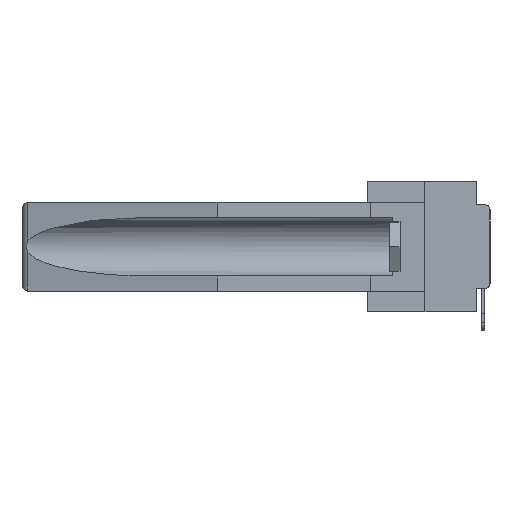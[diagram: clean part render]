
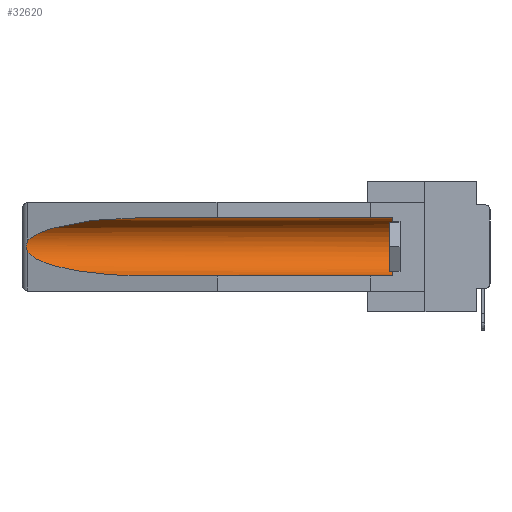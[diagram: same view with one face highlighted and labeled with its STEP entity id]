
A CAD part, left-side view. The second image highlights one B-rep face of the part: STEP entity #32620.
In plain terms, the highlighted cylindrical face has radius 2.857 mm (diameter 5.715 mm), a partial arc.
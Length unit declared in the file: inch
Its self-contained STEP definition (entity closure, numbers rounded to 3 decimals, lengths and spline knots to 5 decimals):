
#6 = CARTESIAN_POINT ( 'NONE',  ( 0.26537, 1.52718, -0.14972 ) ) ;
#1952 = VERTEX_POINT ( 'NONE', #23814 ) ;
#2041 = CARTESIAN_POINT ( 'NONE',  ( 0.155, -0.30754, -0.1715 ) ) ;
#2291 = CARTESIAN_POINT ( 'NONE',  ( 0.26537, 1.52718, -0.19328 ) ) ;
#3107 = VERTEX_POINT ( 'NONE', #19346 ) ;
#3133 = CARTESIAN_POINT ( 'NONE',  ( 0.2673, 1.53269, -0.17917 ) ) ;
#3846 = CARTESIAN_POINT ( 'NONE',  ( 0.21114, 1.30732, -0.284 ) ) ;
#4044 = AXIS2_PLACEMENT_3D ( 'NONE', #2041, #37271, #13783 ) ;
#4428 = VERTEX_POINT ( 'NONE', #21453 ) ;
#6132 = EDGE_CURVE ( 'NONE', #1952, #4428, #11391, .T. ) ;
#6838 = VECTOR ( 'NONE', #12159, 39.37008 ) ;
#6983 = ORIENTED_EDGE ( 'NONE', *, *, #12184, .T. ) ;
#7480 = VERTEX_POINT ( 'NONE', #20083 ) ;
#7540 = FACE_OUTER_BOUND ( 'NONE', #33122, .T. ) ;
#7877 = EDGE_CURVE ( 'NONE', #3107, #36763, #38558, .T. ) ;
#10665 = CARTESIAN_POINT ( 'NONE',  ( 0.25451, 1.48313, -0.09465 ) ) ;
#11354 = CARTESIAN_POINT ( 'NONE',  ( 0.26537, 1.52718, -0.19328 ) ) ;
#11391 = LINE ( 'NONE', #35844, #6838 ) ;
#11836 = AXIS2_PLACEMENT_3D ( 'NONE', #15185, #27341, #18518 ) ;
#12019 = EDGE_CURVE ( 'NONE', #1952, #30955, #21232, .T. ) ;
#12159 = DIRECTION ( 'NONE',  ( 0., 1., 0. ) ) ;
#12184 = EDGE_CURVE ( 'NONE', #36763, #4428, #38624, .T. ) ;
#12767 = DIRECTION ( 'NONE',  ( 0., 1., 0. ) ) ;
#13783 = DIRECTION ( 'NONE',  ( 0., 0., 1. ) ) ;
#13939 = ORIENTED_EDGE ( 'NONE', *, *, #33814, .T. ) ;
#15185 = CARTESIAN_POINT ( 'NONE',  ( 0.155, 0.126, -0.1715 ) ) ;
#15259 = CARTESIAN_POINT ( 'NONE',  ( 0.2675, 1.53308, -0.17534 ) ) ;
#15779 = CARTESIAN_POINT ( 'NONE',  ( 0.155, 1.07973, -0.284 ) ) ;
#16726 = CYLINDRICAL_SURFACE ( 'NONE', #4044, 0.1125 ) ;
#18489 = ORIENTED_EDGE ( 'NONE', *, *, #6132, .F. ) ;
#18514 = CARTESIAN_POINT ( 'NONE',  ( 0.155, 0.126, -0.059 ) ) ;
#18518 = DIRECTION ( 'NONE',  ( 0., 0., 1. ) ) ;
#18631 =( BOUNDED_CURVE ( )  B_SPLINE_CURVE ( 3, ( #28674, #26312, #10665, #19473 ),
 .UNSPECIFIED., .F., .F. ) 
 B_SPLINE_CURVE_WITH_KNOTS ( ( 4, 4 ),
 ( 4.71239, 6.08839 ),
 .UNSPECIFIED. ) 
 CURVE ( )  GEOMETRIC_REPRESENTATION_ITEM ( )  RATIONAL_B_SPLINE_CURVE ( ( 1., 0.848, 0.848, 1. ) ) 
 REPRESENTATION_ITEM ( '' )  );
#19103 = CARTESIAN_POINT ( 'NONE',  ( 0.25451, 1.48313, -0.24835 ) ) ;
#19346 = CARTESIAN_POINT ( 'NONE',  ( 0.26537, 1.52718, -0.14972 ) ) ;
#19473 = CARTESIAN_POINT ( 'NONE',  ( 0.26537, 1.52718, -0.14972 ) ) ;
#20083 = CARTESIAN_POINT ( 'NONE',  ( 0.155, 1.07973, -0.059 ) ) ;
#21232 = CIRCLE ( 'NONE', #11836, 0.1125 ) ;
#21453 = CARTESIAN_POINT ( 'NONE',  ( 0.155, 1.07973, -0.284 ) ) ;
#23814 = CARTESIAN_POINT ( 'NONE',  ( 0.155, 0.126, -0.284 ) ) ;
#23888 = CARTESIAN_POINT ( 'NONE',  ( 0.26654, 1.53092, -0.15636 ) ) ;
#24076 = CARTESIAN_POINT ( 'NONE',  ( 0.2675, 1.53308, -0.16763 ) ) ;
#26312 = CARTESIAN_POINT ( 'NONE',  ( 0.21114, 1.30732, -0.059 ) ) ;
#27208 = CARTESIAN_POINT ( 'NONE',  ( 0.26597, 1.5296, -0.19026 ) ) ;
#27341 = DIRECTION ( 'NONE',  ( 0., -1., 0. ) ) ;
#28674 = CARTESIAN_POINT ( 'NONE',  ( 0.155, 1.07973, -0.059 ) ) ;
#29027 = ORIENTED_EDGE ( 'NONE', *, *, #7877, .T. ) ;
#29837 = ORIENTED_EDGE ( 'NONE', *, *, #12019, .T. ) ;
#30955 = VERTEX_POINT ( 'NONE', #18514 ) ;
#31655 = VECTOR ( 'NONE', #12767, 39.37008 ) ;
#31705 = ORIENTED_EDGE ( 'NONE', *, *, #34112, .T. ) ;
#32315 = CARTESIAN_POINT ( 'NONE',  ( 0.26597, 1.52961, -0.15275 ) ) ;
#32578 = CARTESIAN_POINT ( 'NONE',  ( 0.155, -0.30754, -0.059 ) ) ;
#32620 = ADVANCED_FACE ( 'NONE', ( #7540 ), #16726, .F. ) ;
#33122 = EDGE_LOOP ( 'NONE', ( #13939, #29027, #6983, #18489, #29837, #31705 ) ) ;
#33814 = EDGE_CURVE ( 'NONE', #7480, #3107, #18631, .T. ) ;
#34112 = EDGE_CURVE ( 'NONE', #30955, #7480, #35485, .T. ) ;
#35485 = LINE ( 'NONE', #32578, #31655 ) ;
#35625 = CARTESIAN_POINT ( 'NONE',  ( 0.26655, 1.53094, -0.18657 ) ) ;
#35807 = CARTESIAN_POINT ( 'NONE',  ( 0.2673, 1.5327, -0.16383 ) ) ;
#35844 = CARTESIAN_POINT ( 'NONE',  ( 0.155, -0.30754, -0.284 ) ) ;
#36763 = VERTEX_POINT ( 'NONE', #2291 ) ;
#36907 = CARTESIAN_POINT ( 'NONE',  ( 0.26537, 1.52718, -0.19328 ) ) ;
#37271 = DIRECTION ( 'NONE',  ( 0., 1., 0. ) ) ;
#38558 = B_SPLINE_CURVE_WITH_KNOTS ( 'NONE', 3,
 ( #6, #32315, #23888, #35807, #24076, #15259, #3133, #35625, #27208, #11354 ),
 .UNSPECIFIED., .F., .F.,
 ( 4, 2, 2, 2, 4 ),
 ( 0., 0.00029, 0.00058, 0.00087, 0.00117 ),
 .UNSPECIFIED. ) ;
#38624 =( BOUNDED_CURVE ( )  B_SPLINE_CURVE ( 3, ( #36907, #19103, #3846, #15779 ),
 .UNSPECIFIED., .F., .F. ) 
 B_SPLINE_CURVE_WITH_KNOTS ( ( 4, 4 ),
 ( 0.1948, 1.5708 ),
 .UNSPECIFIED. ) 
 CURVE ( )  GEOMETRIC_REPRESENTATION_ITEM ( )  RATIONAL_B_SPLINE_CURVE ( ( 1., 0.848, 0.848, 1. ) ) 
 REPRESENTATION_ITEM ( '' )  );
